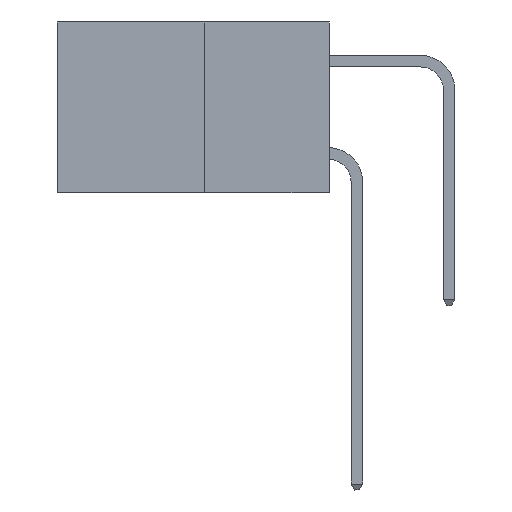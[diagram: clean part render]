
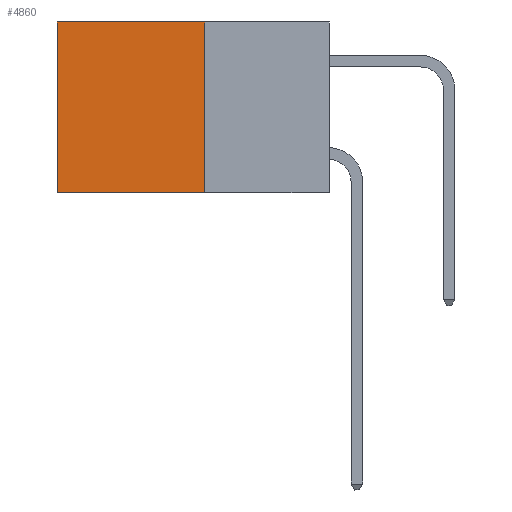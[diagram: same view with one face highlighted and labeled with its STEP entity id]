
A CAD part, left-side view. The second image highlights one B-rep face of the part: STEP entity #4860.
In plain terms, the highlighted planar face has unit normal (-1, 0, 0).
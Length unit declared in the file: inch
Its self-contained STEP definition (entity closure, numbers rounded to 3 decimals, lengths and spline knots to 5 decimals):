
#73 = VERTEX_POINT ( 'NONE', #2272 ) ;
#279 = ORIENTED_EDGE ( 'NONE', *, *, #4159, .T. ) ;
#399 = CARTESIAN_POINT ( 'NONE',  ( 0.277, 0.59, -0.37 ) ) ;
#808 = LINE ( 'NONE', #399, #5791 ) ;
#1335 = LINE ( 'NONE', #2880, #3432 ) ;
#1491 = VECTOR ( 'NONE', #7618, 39.37008 ) ;
#1724 = VERTEX_POINT ( 'NONE', #6384 ) ;
#2255 = ORIENTED_EDGE ( 'NONE', *, *, #2704, .T. ) ;
#2272 = CARTESIAN_POINT ( 'NONE',  ( 0.277, 0.59, -0.37 ) ) ;
#2293 = DIRECTION ( 'NONE',  ( 0., 1., 0. ) ) ;
#2481 = EDGE_CURVE ( 'NONE', #1724, #73, #1335, .T. ) ;
#2570 = CARTESIAN_POINT ( 'NONE',  ( 0.277, 0.27, -0.37 ) ) ;
#2578 = ORIENTED_EDGE ( 'NONE', *, *, #2481, .F. ) ;
#2704 = EDGE_CURVE ( 'NONE', #4866, #8497, #3893, .T. ) ;
#2862 = DIRECTION ( 'NONE',  ( 0., 0., -1. ) ) ;
#2880 = CARTESIAN_POINT ( 'NONE',  ( 0.277, 0.27, -0.37 ) ) ;
#2896 = DIRECTION ( 'NONE',  ( 0., 0., -1. ) ) ;
#3290 = EDGE_LOOP ( 'NONE', ( #279, #2578, #7872, #2255 ) ) ;
#3432 = VECTOR ( 'NONE', #2293, 39.37008 ) ;
#3893 = LINE ( 'NONE', #6503, #1491 ) ;
#4098 = PLANE ( 'NONE',  #5941 ) ;
#4159 = EDGE_CURVE ( 'NONE', #8497, #73, #808, .T. ) ;
#4794 = CARTESIAN_POINT ( 'NONE',  ( 0.277, 0.27, 0. ) ) ;
#4860 = ADVANCED_FACE ( 'NONE', ( #6900 ), #4098, .F. ) ;
#4866 = VERTEX_POINT ( 'NONE', #4794 ) ;
#4941 = EDGE_CURVE ( 'NONE', #4866, #1724, #5166, .T. ) ;
#5166 = LINE ( 'NONE', #2570, #9761 ) ;
#5791 = VECTOR ( 'NONE', #2862, 39.37008 ) ;
#5848 = CARTESIAN_POINT ( 'NONE',  ( 0.277, 0.59, 0. ) ) ;
#5941 = AXIS2_PLACEMENT_3D ( 'NONE', #11044, #12045, #2896 ) ;
#6384 = CARTESIAN_POINT ( 'NONE',  ( 0.277, 0.27, -0.37 ) ) ;
#6503 = CARTESIAN_POINT ( 'NONE',  ( 0.277, 0.27, 0. ) ) ;
#6900 = FACE_OUTER_BOUND ( 'NONE', #3290, .T. ) ;
#7618 = DIRECTION ( 'NONE',  ( 0., 1., 0. ) ) ;
#7872 = ORIENTED_EDGE ( 'NONE', *, *, #4941, .F. ) ;
#8497 = VERTEX_POINT ( 'NONE', #5848 ) ;
#9629 = DIRECTION ( 'NONE',  ( 0., 0., -1. ) ) ;
#9761 = VECTOR ( 'NONE', #9629, 39.37008 ) ;
#11044 = CARTESIAN_POINT ( 'NONE',  ( 0.277, 0.27, -0.37 ) ) ;
#12045 = DIRECTION ( 'NONE',  ( 1., 0., 0. ) ) ;
